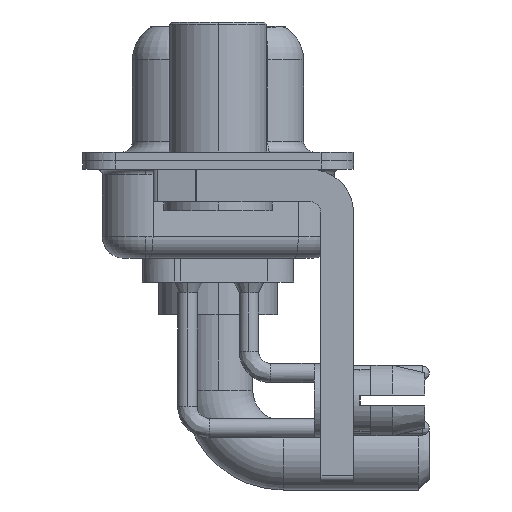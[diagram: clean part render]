
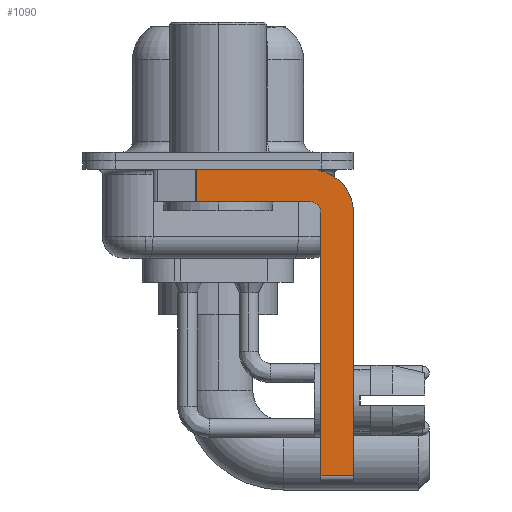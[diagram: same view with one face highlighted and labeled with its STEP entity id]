
A CAD part, left-side view. The second image highlights one B-rep face of the part: STEP entity #1090.
In plain terms, the highlighted planar face has unit normal (-1, 0, 0).
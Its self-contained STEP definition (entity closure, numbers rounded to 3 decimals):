
#16 = VECTOR ( 'NONE', #4854, 1000. ) ;
#1018 = VERTEX_POINT ( 'NONE', #14318 ) ;
#1085 = VECTOR ( 'NONE', #7212, 1000. ) ;
#1090 = ADVANCED_FACE ( 'NONE', ( #8988 ), #8771, .F. ) ;
#2085 = CARTESIAN_POINT ( 'NONE',  ( -2.9, -4.25, -2.4 ) ) ;
#2911 = CARTESIAN_POINT ( 'NONE',  ( -2.9, -4.25, -1.9 ) ) ;
#3051 = DIRECTION ( 'NONE',  ( 0., 0., -1. ) ) ;
#3244 = VECTOR ( 'NONE', #14479, 1000. ) ;
#3275 = CARTESIAN_POINT ( 'NONE',  ( -2.9, 0.978, -1.9 ) ) ;
#3653 = VERTEX_POINT ( 'NONE', #21831 ) ;
#3909 = DIRECTION ( 'NONE',  ( -1., 0., 0. ) ) ;
#4138 = ORIENTED_EDGE ( 'NONE', *, *, #21715, .F. ) ;
#4658 = AXIS2_PLACEMENT_3D ( 'NONE', #17810, #3909, #6015 ) ;
#4854 = DIRECTION ( 'NONE',  ( 0., 0., -1. ) ) ;
#4942 = ORIENTED_EDGE ( 'NONE', *, *, #9337, .F. ) ;
#5192 = LINE ( 'NONE', #18773, #18527 ) ;
#5678 = CARTESIAN_POINT ( 'NONE',  ( -2.9, 3., -0.4 ) ) ;
#5686 = CARTESIAN_POINT ( 'NONE',  ( -2.9, -4.25, -1.9 ) ) ;
#6015 = DIRECTION ( 'NONE',  ( 0., 0., 1. ) ) ;
#6346 = VECTOR ( 'NONE', #12480, 1000. ) ;
#6395 = DIRECTION ( 'NONE',  ( 1., 0., 0. ) ) ;
#7027 = CARTESIAN_POINT ( 'NONE',  ( -2.9, 0.978, -1.9 ) ) ;
#7075 = VERTEX_POINT ( 'NONE', #14920 ) ;
#7212 = DIRECTION ( 'NONE',  ( 0., -1., 0. ) ) ;
#7877 = EDGE_LOOP ( 'NONE', ( #19630, #16943, #16452, #21394, #4942, #13692, #4138, #16477 ) ) ;
#8122 = AXIS2_PLACEMENT_3D ( 'NONE', #14864, #6395, #13191 ) ;
#8201 = EDGE_CURVE ( 'NONE', #1018, #7075, #17008, .T. ) ;
#8771 = PLANE ( 'NONE',  #16169 ) ;
#8862 = CARTESIAN_POINT ( 'NONE',  ( -2.9, -4.75, -2.4 ) ) ;
#8988 = FACE_OUTER_BOUND ( 'NONE', #7877, .T. ) ;
#9280 = VECTOR ( 'NONE', #3051, 1000. ) ;
#9337 = EDGE_CURVE ( 'NONE', #19862, #17138, #5192, .T. ) ;
#10002 = CIRCLE ( 'NONE', #4658, 0.5 ) ;
#10781 = LINE ( 'NONE', #17560, #1085 ) ;
#11204 = CARTESIAN_POINT ( 'NONE',  ( -2.9, -6.25, -2.4 ) ) ;
#12480 = DIRECTION ( 'NONE',  ( 0., -1., 0. ) ) ;
#13053 = VERTEX_POINT ( 'NONE', #16723 ) ;
#13191 = DIRECTION ( 'NONE',  ( 0., 0., -1. ) ) ;
#13692 = ORIENTED_EDGE ( 'NONE', *, *, #19792, .T. ) ;
#14144 = LINE ( 'NONE', #5686, #3244 ) ;
#14318 = CARTESIAN_POINT ( 'NONE',  ( -2.9, -4.25, -0.4 ) ) ;
#14479 = DIRECTION ( 'NONE',  ( 0., 1., 0. ) ) ;
#14864 = CARTESIAN_POINT ( 'NONE',  ( -2.9, -4.25, -2.4 ) ) ;
#14920 = CARTESIAN_POINT ( 'NONE',  ( -2.9, -6.25, -2.4 ) ) ;
#15080 = LINE ( 'NONE', #3275, #9280 ) ;
#15775 = DIRECTION ( 'NONE',  ( 1., 0., 0. ) ) ;
#15963 = VERTEX_POINT ( 'NONE', #7027 ) ;
#16169 = AXIS2_PLACEMENT_3D ( 'NONE', #2085, #15775, #17654 ) ;
#16181 = EDGE_CURVE ( 'NONE', #13053, #1018, #21033, .T. ) ;
#16452 = ORIENTED_EDGE ( 'NONE', *, *, #20223, .F. ) ;
#16477 = ORIENTED_EDGE ( 'NONE', *, *, #8201, .F. ) ;
#16723 = CARTESIAN_POINT ( 'NONE',  ( -2.9, 0.978, -0.4 ) ) ;
#16742 = CARTESIAN_POINT ( 'NONE',  ( -2.9, -4.75, -14.55 ) ) ;
#16943 = ORIENTED_EDGE ( 'NONE', *, *, #20351, .T. ) ;
#17008 = CIRCLE ( 'NONE', #8122, 2. ) ;
#17138 = VERTEX_POINT ( 'NONE', #8862 ) ;
#17560 = CARTESIAN_POINT ( 'NONE',  ( -2.9, -4.25, -14.55 ) ) ;
#17654 = DIRECTION ( 'NONE',  ( 0., 0., -1. ) ) ;
#17810 = CARTESIAN_POINT ( 'NONE',  ( -2.9, -4.25, -2.4 ) ) ;
#18527 = VECTOR ( 'NONE', #18885, 1000. ) ;
#18624 = VERTEX_POINT ( 'NONE', #2911 ) ;
#18773 = CARTESIAN_POINT ( 'NONE',  ( -2.9, -4.75, -14.8 ) ) ;
#18885 = DIRECTION ( 'NONE',  ( 0., 0., 1. ) ) ;
#19630 = ORIENTED_EDGE ( 'NONE', *, *, #16181, .F. ) ;
#19792 = EDGE_CURVE ( 'NONE', #19862, #3653, #10781, .T. ) ;
#19862 = VERTEX_POINT ( 'NONE', #16742 ) ;
#20223 = EDGE_CURVE ( 'NONE', #18624, #15963, #14144, .T. ) ;
#20254 = EDGE_CURVE ( 'NONE', #17138, #18624, #10002, .T. ) ;
#20351 = EDGE_CURVE ( 'NONE', #13053, #15963, #15080, .T. ) ;
#21033 = LINE ( 'NONE', #5678, #6346 ) ;
#21316 = LINE ( 'NONE', #11204, #16 ) ;
#21394 = ORIENTED_EDGE ( 'NONE', *, *, #20254, .F. ) ;
#21715 = EDGE_CURVE ( 'NONE', #7075, #3653, #21316, .T. ) ;
#21831 = CARTESIAN_POINT ( 'NONE',  ( -2.9, -6.25, -14.55 ) ) ;
